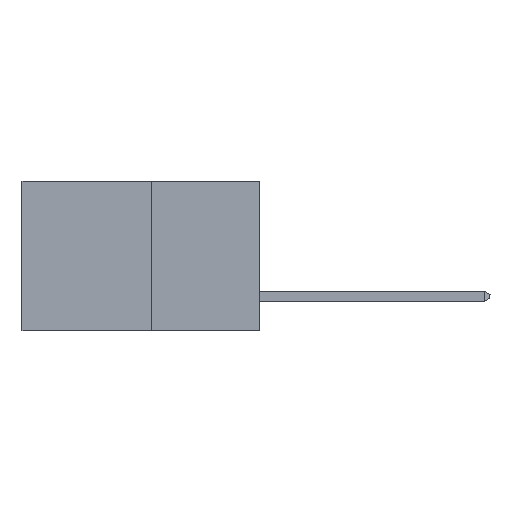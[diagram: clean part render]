
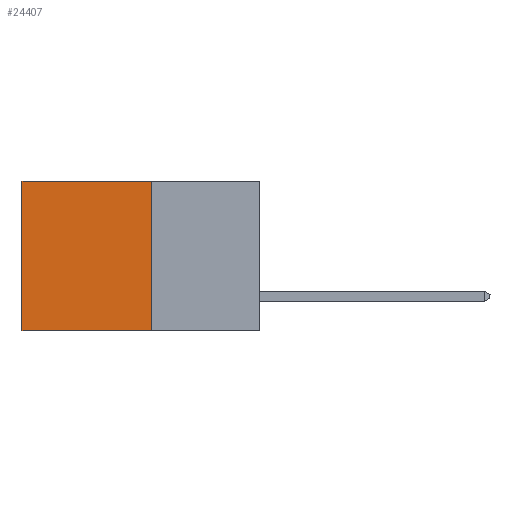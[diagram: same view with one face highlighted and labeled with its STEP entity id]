
A CAD part, left-side view. The second image highlights one B-rep face of the part: STEP entity #24407.
In plain terms, the highlighted planar face has unit normal (-1, 0, 0).
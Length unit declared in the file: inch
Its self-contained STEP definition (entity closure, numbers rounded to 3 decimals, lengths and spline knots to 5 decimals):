
#3427 = ORIENTED_EDGE ( 'NONE', *, *, #19678, .F. ) ;
#3687 = VECTOR ( 'NONE', #25279, 39.37008 ) ;
#4966 = LINE ( 'NONE', #10118, #27838 ) ;
#5337 = VECTOR ( 'NONE', #17524, 39.37008 ) ;
#5430 = PLANE ( 'NONE',  #27287 ) ;
#5912 = CARTESIAN_POINT ( 'NONE',  ( 0.277, 0.27, 0. ) ) ;
#7124 = CARTESIAN_POINT ( 'NONE',  ( 0.277, 0.59, -0.37 ) ) ;
#7389 = CARTESIAN_POINT ( 'NONE',  ( 0.277, 0.27, -0.37 ) ) ;
#7585 = VERTEX_POINT ( 'NONE', #19766 ) ;
#10032 = DIRECTION ( 'NONE',  ( 0., 0., -1. ) ) ;
#10118 = CARTESIAN_POINT ( 'NONE',  ( 0.277, 0.27, -0.37 ) ) ;
#10669 = VECTOR ( 'NONE', #14079, 39.37008 ) ;
#12085 = CARTESIAN_POINT ( 'NONE',  ( 0.277, 0.27, 0. ) ) ;
#12417 = ORIENTED_EDGE ( 'NONE', *, *, #22666, .T. ) ;
#14079 = DIRECTION ( 'NONE',  ( 0., 1., 0. ) ) ;
#15619 = ORIENTED_EDGE ( 'NONE', *, *, #23576, .F. ) ;
#17507 = ORIENTED_EDGE ( 'NONE', *, *, #28473, .T. ) ;
#17524 = DIRECTION ( 'NONE',  ( 0., 1., 0. ) ) ;
#17737 = CARTESIAN_POINT ( 'NONE',  ( 0.277, 0.59, 0. ) ) ;
#17809 = FACE_OUTER_BOUND ( 'NONE', #23956, .T. ) ;
#19678 = EDGE_CURVE ( 'NONE', #25873, #25840, #4966, .T. ) ;
#19766 = CARTESIAN_POINT ( 'NONE',  ( 0.277, 0.59, -0.37 ) ) ;
#21399 = CARTESIAN_POINT ( 'NONE',  ( 0.277, 0.27, -0.37 ) ) ;
#22666 = EDGE_CURVE ( 'NONE', #25873, #28231, #29636, .T. ) ;
#23170 = CARTESIAN_POINT ( 'NONE',  ( 0.277, 0.27, -0.37 ) ) ;
#23576 = EDGE_CURVE ( 'NONE', #25840, #7585, #28878, .T. ) ;
#23717 = DIRECTION ( 'NONE',  ( 1., 0., 0. ) ) ;
#23956 = EDGE_LOOP ( 'NONE', ( #17507, #15619, #3427, #12417 ) ) ;
#24407 = ADVANCED_FACE ( 'NONE', ( #17809 ), #5430, .F. ) ;
#25279 = DIRECTION ( 'NONE',  ( 0., 0., -1. ) ) ;
#25840 = VERTEX_POINT ( 'NONE', #7389 ) ;
#25873 = VERTEX_POINT ( 'NONE', #12085 ) ;
#26080 = DIRECTION ( 'NONE',  ( 0., 0., -1. ) ) ;
#27287 = AXIS2_PLACEMENT_3D ( 'NONE', #21399, #23717, #10032 ) ;
#27838 = VECTOR ( 'NONE', #26080, 39.37008 ) ;
#28231 = VERTEX_POINT ( 'NONE', #17737 ) ;
#28473 = EDGE_CURVE ( 'NONE', #28231, #7585, #28729, .T. ) ;
#28729 = LINE ( 'NONE', #7124, #3687 ) ;
#28878 = LINE ( 'NONE', #23170, #10669 ) ;
#29636 = LINE ( 'NONE', #5912, #5337 ) ;
